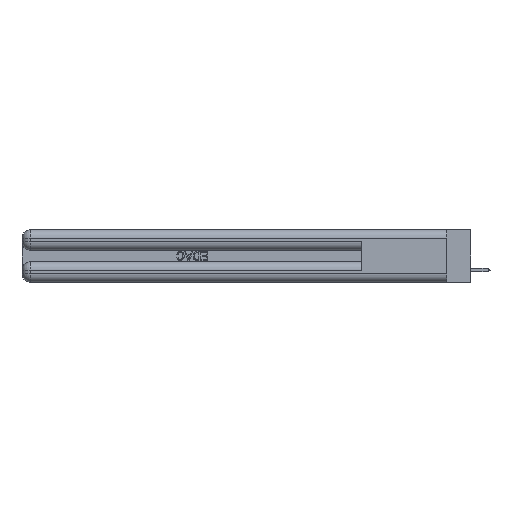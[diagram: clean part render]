
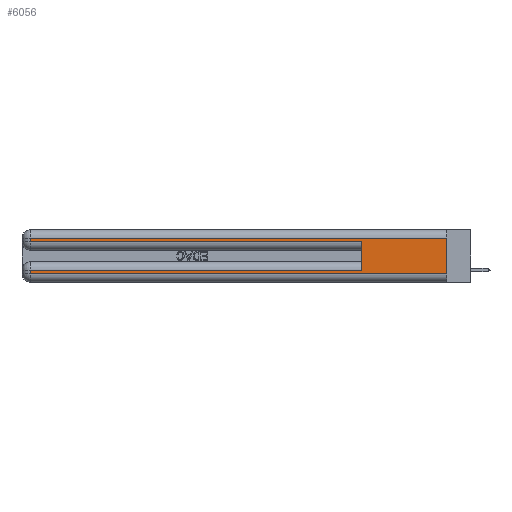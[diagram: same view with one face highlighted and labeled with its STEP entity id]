
A CAD part, left-side view. The second image highlights one B-rep face of the part: STEP entity #6056.
In plain terms, the highlighted planar face has unit normal (-1, 0, 0).
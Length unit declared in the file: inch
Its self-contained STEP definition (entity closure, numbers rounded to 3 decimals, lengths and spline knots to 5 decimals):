
#625 = CARTESIAN_POINT ( 'NONE',  ( 0., 0., 0.37 ) ) ;
#785 = CARTESIAN_POINT ( 'NONE',  ( 0., 0., 0.085 ) ) ;
#910 = DIRECTION ( 'NONE',  ( 0., -1., 0. ) ) ;
#1023 = LINE ( 'NONE', #785, #15701 ) ;
#2157 = VECTOR ( 'NONE', #910, 39.37008 ) ;
#2655 = PLANE ( 'NONE',  #25295 ) ;
#3827 = CARTESIAN_POINT ( 'NONE',  ( 0., 2.94, 0.31 ) ) ;
#4192 = CARTESIAN_POINT ( 'NONE',  ( 0., 2.94, 0.085 ) ) ;
#4449 = EDGE_CURVE ( 'NONE', #28088, #5355, #1023, .T. ) ;
#4867 = DIRECTION ( 'NONE',  ( 0., 0., -1. ) ) ;
#4893 = VERTEX_POINT ( 'NONE', #25366 ) ;
#5355 = VERTEX_POINT ( 'NONE', #4192 ) ;
#5605 = ORIENTED_EDGE ( 'NONE', *, *, #34601, .F. ) ;
#5642 = VERTEX_POINT ( 'NONE', #18331 ) ;
#5699 = ORIENTED_EDGE ( 'NONE', *, *, #33155, .T. ) ;
#5903 = VECTOR ( 'NONE', #13337, 39.37008 ) ;
#6056 = ADVANCED_FACE ( 'NONE', ( #30820 ), #2655, .F. ) ;
#6071 = ORIENTED_EDGE ( 'NONE', *, *, #8732, .F. ) ;
#6770 = VECTOR ( 'NONE', #28328, 39.37008 ) ;
#7075 = CARTESIAN_POINT ( 'NONE',  ( 0., 2.94, 0.06 ) ) ;
#8732 = EDGE_CURVE ( 'NONE', #28088, #32431, #21413, .T. ) ;
#9751 = VECTOR ( 'NONE', #31511, 39.37008 ) ;
#10199 = ORIENTED_EDGE ( 'NONE', *, *, #22332, .T. ) ;
#11272 = LINE ( 'NONE', #28668, #16135 ) ;
#11534 = CARTESIAN_POINT ( 'NONE',  ( 0., 0.6, 0.145 ) ) ;
#12180 = CARTESIAN_POINT ( 'NONE',  ( 0., 0.6, 0.285 ) ) ;
#12263 = CARTESIAN_POINT ( 'NONE',  ( 0., 0., 0.06 ) ) ;
#12900 = EDGE_LOOP ( 'NONE', ( #5605, #29214, #10199, #16563, #6071, #36297, #34982, #5699 ) ) ;
#13337 = DIRECTION ( 'NONE',  ( 0., 0., -1. ) ) ;
#13450 = CARTESIAN_POINT ( 'NONE',  ( 0., 2.94, 0.285 ) ) ;
#14316 = CARTESIAN_POINT ( 'NONE',  ( 0., 0., 0.285 ) ) ;
#14985 = DIRECTION ( 'NONE',  ( 0., 1., 0. ) ) ;
#15701 = VECTOR ( 'NONE', #14985, 39.37008 ) ;
#16135 = VECTOR ( 'NONE', #17316, 39.37008 ) ;
#16563 = ORIENTED_EDGE ( 'NONE', *, *, #23951, .T. ) ;
#17316 = DIRECTION ( 'NONE',  ( 0., 1., 0. ) ) ;
#18165 = LINE ( 'NONE', #12263, #2157 ) ;
#18331 = CARTESIAN_POINT ( 'NONE',  ( 0., 0., 0.06 ) ) ;
#18772 = LINE ( 'NONE', #30402, #5903 ) ;
#19366 = DIRECTION ( 'NONE',  ( 0., 0., -1. ) ) ;
#21413 = LINE ( 'NONE', #11534, #6770 ) ;
#21954 = EDGE_CURVE ( 'NONE', #4893, #32521, #11272, .T. ) ;
#22332 = EDGE_CURVE ( 'NONE', #32521, #31454, #31741, .T. ) ;
#22344 = EDGE_CURVE ( 'NONE', #5355, #26227, #18772, .T. ) ;
#23394 = VECTOR ( 'NONE', #19366, 39.37008 ) ;
#23951 = EDGE_CURVE ( 'NONE', #31454, #32431, #28913, .T. ) ;
#24141 = VECTOR ( 'NONE', #4867, 39.37008 ) ;
#25295 = AXIS2_PLACEMENT_3D ( 'NONE', #625, #27160, #30029 ) ;
#25366 = CARTESIAN_POINT ( 'NONE',  ( 0., 0., 0.31 ) ) ;
#26227 = VERTEX_POINT ( 'NONE', #7075 ) ;
#27160 = DIRECTION ( 'NONE',  ( 1., 0., 0. ) ) ;
#28088 = VERTEX_POINT ( 'NONE', #29824 ) ;
#28328 = DIRECTION ( 'NONE',  ( 0., 0., 1. ) ) ;
#28340 = CARTESIAN_POINT ( 'NONE',  ( 0., 0., 0.37 ) ) ;
#28668 = CARTESIAN_POINT ( 'NONE',  ( 0., 0., 0.31 ) ) ;
#28913 = LINE ( 'NONE', #14316, #9751 ) ;
#29214 = ORIENTED_EDGE ( 'NONE', *, *, #21954, .T. ) ;
#29824 = CARTESIAN_POINT ( 'NONE',  ( 0., 0.6, 0.085 ) ) ;
#30029 = DIRECTION ( 'NONE',  ( 0., 0., -1. ) ) ;
#30402 = CARTESIAN_POINT ( 'NONE',  ( 0., 2.94, 0.37 ) ) ;
#30820 = FACE_OUTER_BOUND ( 'NONE', #12900, .T. ) ;
#30990 = LINE ( 'NONE', #28340, #23394 ) ;
#31454 = VERTEX_POINT ( 'NONE', #13450 ) ;
#31511 = DIRECTION ( 'NONE',  ( 0., -1., 0. ) ) ;
#31741 = LINE ( 'NONE', #35889, #24141 ) ;
#32431 = VERTEX_POINT ( 'NONE', #12180 ) ;
#32521 = VERTEX_POINT ( 'NONE', #3827 ) ;
#33155 = EDGE_CURVE ( 'NONE', #26227, #5642, #18165, .T. ) ;
#34601 = EDGE_CURVE ( 'NONE', #4893, #5642, #30990, .T. ) ;
#34982 = ORIENTED_EDGE ( 'NONE', *, *, #22344, .T. ) ;
#35889 = CARTESIAN_POINT ( 'NONE',  ( 0., 2.94, 0.37 ) ) ;
#36297 = ORIENTED_EDGE ( 'NONE', *, *, #4449, .T. ) ;
